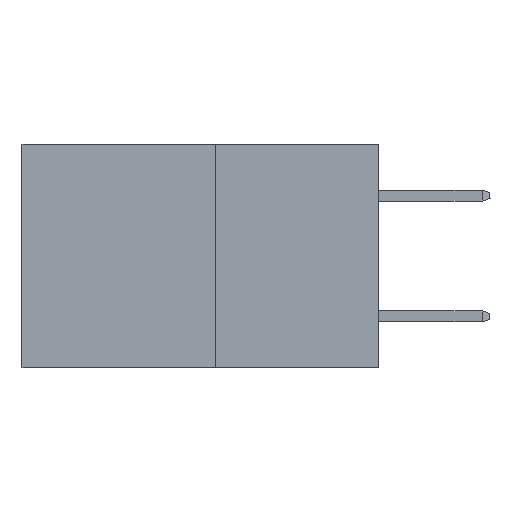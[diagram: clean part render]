
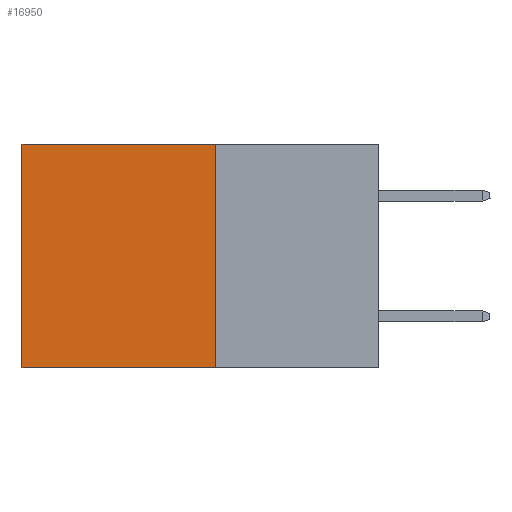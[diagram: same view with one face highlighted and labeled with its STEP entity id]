
A CAD part, left-side view. The second image highlights one B-rep face of the part: STEP entity #16950.
In plain terms, the highlighted planar face has unit normal (-1, 0, 0).
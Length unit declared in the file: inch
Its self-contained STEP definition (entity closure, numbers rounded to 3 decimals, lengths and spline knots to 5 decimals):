
#777 = VECTOR ( 'NONE', #20644, 39.37008 ) ;
#3084 = VECTOR ( 'NONE', #15744, 39.37008 ) ;
#3628 = LINE ( 'NONE', #16507, #3084 ) ;
#4508 = EDGE_CURVE ( 'NONE', #17889, #15819, #12023, .T. ) ;
#5228 = CARTESIAN_POINT ( 'NONE',  ( 0.277, 0.59, 0. ) ) ;
#5927 = EDGE_CURVE ( 'NONE', #15819, #10511, #18880, .T. ) ;
#8269 = AXIS2_PLACEMENT_3D ( 'NONE', #17996, #18158, #18209 ) ;
#9134 = CARTESIAN_POINT ( 'NONE',  ( 0.277, 0.27, 0. ) ) ;
#9810 = DIRECTION ( 'NONE',  ( 0., 1., 0. ) ) ;
#10235 = VERTEX_POINT ( 'NONE', #5228 ) ;
#10346 = EDGE_LOOP ( 'NONE', ( #16987, #18820, #13250, #15660 ) ) ;
#10511 = VERTEX_POINT ( 'NONE', #17016 ) ;
#10983 = CARTESIAN_POINT ( 'NONE',  ( 0.277, 0.27, -0.37 ) ) ;
#11152 = EDGE_CURVE ( 'NONE', #10235, #10511, #3628, .T. ) ;
#12023 = LINE ( 'NONE', #13015, #21051 ) ;
#13015 = CARTESIAN_POINT ( 'NONE',  ( 0.277, 0.27, -0.37 ) ) ;
#13183 = VECTOR ( 'NONE', #9810, 39.37008 ) ;
#13250 = ORIENTED_EDGE ( 'NONE', *, *, #4508, .F. ) ;
#13285 = DIRECTION ( 'NONE',  ( 0., 0., -1. ) ) ;
#15228 = FACE_OUTER_BOUND ( 'NONE', #10346, .T. ) ;
#15660 = ORIENTED_EDGE ( 'NONE', *, *, #20911, .T. ) ;
#15744 = DIRECTION ( 'NONE',  ( 0., 0., -1. ) ) ;
#15819 = VERTEX_POINT ( 'NONE', #10983 ) ;
#16507 = CARTESIAN_POINT ( 'NONE',  ( 0.277, 0.59, -0.37 ) ) ;
#16950 = ADVANCED_FACE ( 'NONE', ( #15228 ), #18137, .F. ) ;
#16987 = ORIENTED_EDGE ( 'NONE', *, *, #11152, .T. ) ;
#17016 = CARTESIAN_POINT ( 'NONE',  ( 0.277, 0.59, -0.37 ) ) ;
#17442 = CARTESIAN_POINT ( 'NONE',  ( 0.277, 0.27, -0.37 ) ) ;
#17889 = VERTEX_POINT ( 'NONE', #9134 ) ;
#17996 = CARTESIAN_POINT ( 'NONE',  ( 0.277, 0.27, -0.37 ) ) ;
#18137 = PLANE ( 'NONE',  #8269 ) ;
#18158 = DIRECTION ( 'NONE',  ( 1., 0., 0. ) ) ;
#18209 = DIRECTION ( 'NONE',  ( 0., 0., -1. ) ) ;
#18820 = ORIENTED_EDGE ( 'NONE', *, *, #5927, .F. ) ;
#18880 = LINE ( 'NONE', #17442, #777 ) ;
#19996 = CARTESIAN_POINT ( 'NONE',  ( 0.277, 0.27, 0. ) ) ;
#20644 = DIRECTION ( 'NONE',  ( 0., 1., 0. ) ) ;
#20911 = EDGE_CURVE ( 'NONE', #17889, #10235, #21145, .T. ) ;
#21051 = VECTOR ( 'NONE', #13285, 39.37008 ) ;
#21145 = LINE ( 'NONE', #19996, #13183 ) ;
